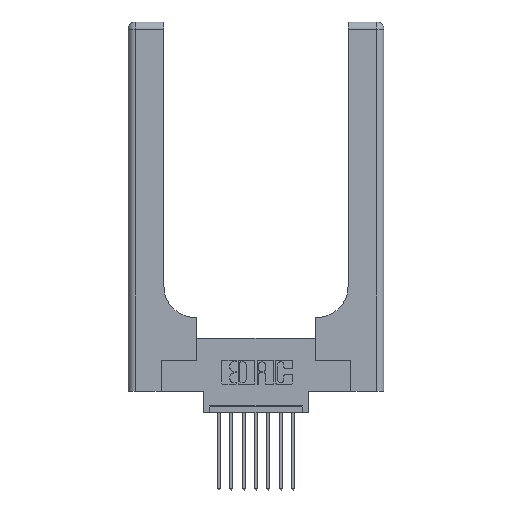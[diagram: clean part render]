
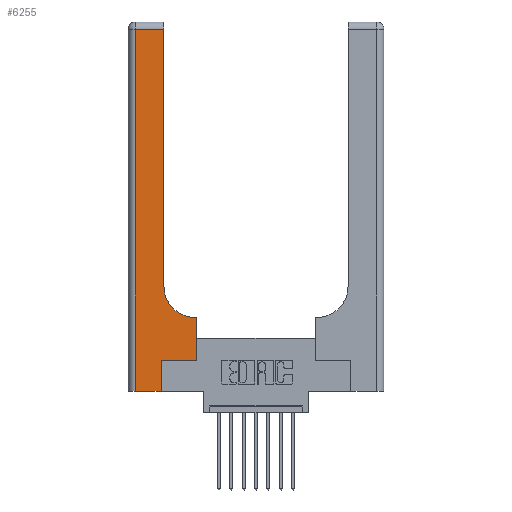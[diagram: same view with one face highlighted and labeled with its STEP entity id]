
A CAD part, top view. The second image highlights one B-rep face of the part: STEP entity #6255.
In plain terms, the highlighted planar face has unit normal (0, 0, 1).
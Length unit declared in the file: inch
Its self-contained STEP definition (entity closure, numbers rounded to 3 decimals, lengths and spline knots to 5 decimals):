
#84 = CARTESIAN_POINT ( 'NONE',  ( 0.2915, 0.85, 0.37 ) ) ;
#195 = EDGE_CURVE ( 'NONE', #2919, #3677, #6805, .T. ) ;
#364 = ORIENTED_EDGE ( 'NONE', *, *, #5998, .T. ) ;
#544 = FACE_OUTER_BOUND ( 'NONE', #5114, .T. ) ;
#549 = DIRECTION ( 'NONE',  ( 0., 0., -1. ) ) ;
#911 = VECTOR ( 'NONE', #14361, 39.37008 ) ;
#1120 = VERTEX_POINT ( 'NONE', #9091 ) ;
#1386 = EDGE_CURVE ( 'NONE', #14715, #8551, #4033, .T. ) ;
#2117 = ORIENTED_EDGE ( 'NONE', *, *, #12470, .T. ) ;
#2218 = EDGE_CURVE ( 'NONE', #14969, #14715, #10427, .T. ) ;
#2466 = LINE ( 'NONE', #11056, #5237 ) ;
#2491 = EDGE_CURVE ( 'NONE', #3677, #13485, #2877, .T. ) ;
#2809 = DIRECTION ( 'NONE',  ( 0., -1., 0. ) ) ;
#2877 = LINE ( 'NONE', #9511, #12671 ) ;
#2919 = VERTEX_POINT ( 'NONE', #9617 ) ;
#3652 = DIRECTION ( 'NONE',  ( 0., 1., 0. ) ) ;
#3677 = VERTEX_POINT ( 'NONE', #8688 ) ;
#3874 = CIRCLE ( 'NONE', #4597, 0.25 ) ;
#4033 = LINE ( 'NONE', #7463, #911 ) ;
#4065 = VECTOR ( 'NONE', #3652, 39.37008 ) ;
#4350 = ORIENTED_EDGE ( 'NONE', *, *, #7687, .T. ) ;
#4524 = DIRECTION ( 'NONE',  ( 0., 0., -1. ) ) ;
#4597 = AXIS2_PLACEMENT_3D ( 'NONE', #14198, #4524, #4670 ) ;
#4670 = DIRECTION ( 'NONE',  ( 1., 0., 0. ) ) ;
#4849 = CARTESIAN_POINT ( 'NONE',  ( 0.5585, 0.25, 0.37 ) ) ;
#5114 = EDGE_LOOP ( 'NONE', ( #2117, #10639, #4350, #7950, #11050, #364, #6683, #15083, #5770 ) ) ;
#5237 = VECTOR ( 'NONE', #9742, 39.37008 ) ;
#5418 = DIRECTION ( 'NONE',  ( -1., 0., 0. ) ) ;
#5487 = VECTOR ( 'NONE', #2809, 39.37008 ) ;
#5770 = ORIENTED_EDGE ( 'NONE', *, *, #12177, .T. ) ;
#5998 = EDGE_CURVE ( 'NONE', #8551, #2919, #10837, .T. ) ;
#6255 = ADVANCED_FACE ( 'NONE', ( #544 ), #12396, .F. ) ;
#6683 = ORIENTED_EDGE ( 'NONE', *, *, #195, .T. ) ;
#6686 = CARTESIAN_POINT ( 'NONE',  ( 0., 0., 0.37 ) ) ;
#6805 = LINE ( 'NONE', #4849, #4065 ) ;
#7009 = VERTEX_POINT ( 'NONE', #84 ) ;
#7453 = VERTEX_POINT ( 'NONE', #11830 ) ;
#7463 = CARTESIAN_POINT ( 'NONE',  ( 0.269, 0., 0.37 ) ) ;
#7551 = DIRECTION ( 'NONE',  ( -1., 0., 0. ) ) ;
#7594 = DIRECTION ( 'NONE',  ( -1., 0., 0. ) ) ;
#7687 = EDGE_CURVE ( 'NONE', #1120, #14969, #14546, .T. ) ;
#7950 = ORIENTED_EDGE ( 'NONE', *, *, #2218, .T. ) ;
#8551 = VERTEX_POINT ( 'NONE', #8677 ) ;
#8677 = CARTESIAN_POINT ( 'NONE',  ( 0.269, 0.25, 0.37 ) ) ;
#8688 = CARTESIAN_POINT ( 'NONE',  ( 0.5585, 0.6, 0.37 ) ) ;
#9091 = CARTESIAN_POINT ( 'NONE',  ( 0.06, 2.94, 0.37 ) ) ;
#9511 = CARTESIAN_POINT ( 'NONE',  ( 0.2915, 0.6, 0.37 ) ) ;
#9617 = CARTESIAN_POINT ( 'NONE',  ( 0.5585, 0.25, 0.37 ) ) ;
#9713 = VECTOR ( 'NONE', #11877, 39.37008 ) ;
#9742 = DIRECTION ( 'NONE',  ( 0., 1., 0. ) ) ;
#9825 = CARTESIAN_POINT ( 'NONE',  ( 0.06, 0., 0.37 ) ) ;
#9839 = EDGE_CURVE ( 'NONE', #7453, #1120, #14694, .T. ) ;
#9848 = CARTESIAN_POINT ( 'NONE',  ( 0.06, 3., 0.37 ) ) ;
#10427 = LINE ( 'NONE', #6686, #11925 ) ;
#10444 = CARTESIAN_POINT ( 'NONE',  ( 0.269, 0., 0.37 ) ) ;
#10585 = CARTESIAN_POINT ( 'NONE',  ( 0.5415, 0.6, 0.37 ) ) ;
#10639 = ORIENTED_EDGE ( 'NONE', *, *, #9839, .T. ) ;
#10837 = LINE ( 'NONE', #13187, #9713 ) ;
#11050 = ORIENTED_EDGE ( 'NONE', *, *, #1386, .T. ) ;
#11056 = CARTESIAN_POINT ( 'NONE',  ( 0.2915, 3., 0.37 ) ) ;
#11057 = AXIS2_PLACEMENT_3D ( 'NONE', #13456, #549, #7594 ) ;
#11279 = CARTESIAN_POINT ( 'NONE',  ( 0., 2.94, 0.37 ) ) ;
#11502 = VECTOR ( 'NONE', #5418, 39.37008 ) ;
#11830 = CARTESIAN_POINT ( 'NONE',  ( 0.2915, 2.94, 0.37 ) ) ;
#11877 = DIRECTION ( 'NONE',  ( 1., 0., 0. ) ) ;
#11925 = VECTOR ( 'NONE', #12855, 39.37008 ) ;
#12177 = EDGE_CURVE ( 'NONE', #13485, #7009, #3874, .T. ) ;
#12396 = PLANE ( 'NONE',  #11057 ) ;
#12470 = EDGE_CURVE ( 'NONE', #7009, #7453, #2466, .T. ) ;
#12671 = VECTOR ( 'NONE', #7551, 39.37008 ) ;
#12855 = DIRECTION ( 'NONE',  ( 1., 0., 0. ) ) ;
#13187 = CARTESIAN_POINT ( 'NONE',  ( 0.269, 0.25, 0.37 ) ) ;
#13456 = CARTESIAN_POINT ( 'NONE',  ( 0., 3., 0.37 ) ) ;
#13485 = VERTEX_POINT ( 'NONE', #10585 ) ;
#14198 = CARTESIAN_POINT ( 'NONE',  ( 0.5415, 0.85, 0.37 ) ) ;
#14361 = DIRECTION ( 'NONE',  ( 0., 1., 0. ) ) ;
#14546 = LINE ( 'NONE', #9848, #5487 ) ;
#14694 = LINE ( 'NONE', #11279, #11502 ) ;
#14715 = VERTEX_POINT ( 'NONE', #10444 ) ;
#14969 = VERTEX_POINT ( 'NONE', #9825 ) ;
#15083 = ORIENTED_EDGE ( 'NONE', *, *, #2491, .T. ) ;
